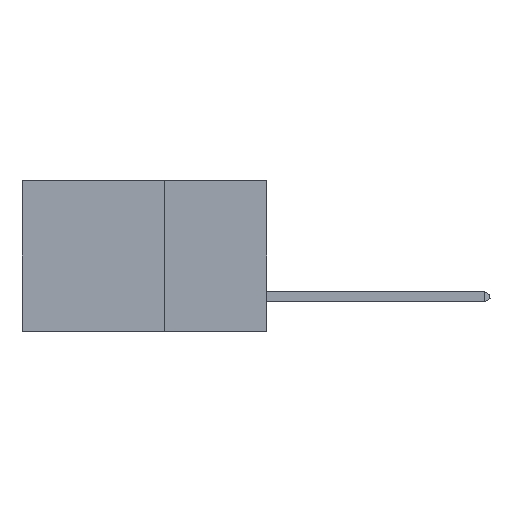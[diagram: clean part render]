
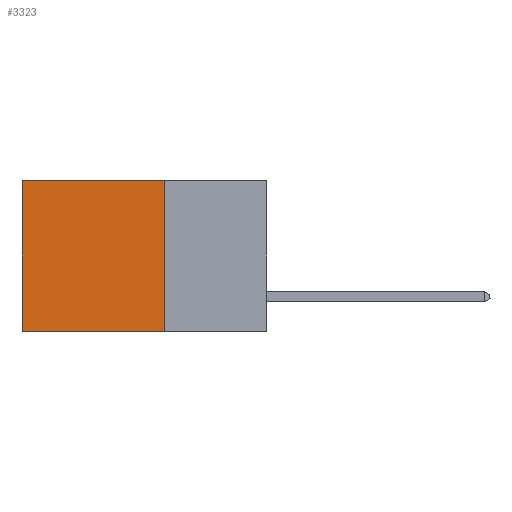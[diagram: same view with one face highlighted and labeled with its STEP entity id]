
A CAD part, left-side view. The second image highlights one B-rep face of the part: STEP entity #3323.
In plain terms, the highlighted planar face has unit normal (-1, 0, 0).
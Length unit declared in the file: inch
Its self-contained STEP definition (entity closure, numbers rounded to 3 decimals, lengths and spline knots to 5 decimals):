
#130 = ORIENTED_EDGE ( 'NONE', *, *, #22767, .F. ) ;
#2065 = CARTESIAN_POINT ( 'NONE',  ( 0.2875, 0.25, 0. ) ) ;
#2497 = DIRECTION ( 'NONE',  ( 0., 1., 0. ) ) ;
#3039 = VERTEX_POINT ( 'NONE', #33966 ) ;
#3323 = ADVANCED_FACE ( 'NONE', ( #24807 ), #29328, .F. ) ;
#4617 = LINE ( 'NONE', #5900, #30110 ) ;
#5057 = ORIENTED_EDGE ( 'NONE', *, *, #29074, .F. ) ;
#5900 = CARTESIAN_POINT ( 'NONE',  ( 0.2875, 0.25, 0. ) ) ;
#6223 = VERTEX_POINT ( 'NONE', #16613 ) ;
#7094 = CARTESIAN_POINT ( 'NONE',  ( 0.2875, 0.25, 0. ) ) ;
#10173 = CARTESIAN_POINT ( 'NONE',  ( 0.2875, 0.6, 0. ) ) ;
#11551 = AXIS2_PLACEMENT_3D ( 'NONE', #29698, #20907, #32664 ) ;
#12199 = LINE ( 'NONE', #32930, #18725 ) ;
#16613 = CARTESIAN_POINT ( 'NONE',  ( 0.2875, 0.6, -0.37 ) ) ;
#18725 = VECTOR ( 'NONE', #32424, 39.37008 ) ;
#19114 = DIRECTION ( 'NONE',  ( 0., 0., -1. ) ) ;
#20099 = LINE ( 'NONE', #2065, #28431 ) ;
#20907 = DIRECTION ( 'NONE',  ( 1., 0., 0. ) ) ;
#22478 = CARTESIAN_POINT ( 'NONE',  ( 0.2875, 0.6, 0. ) ) ;
#22767 = EDGE_CURVE ( 'NONE', #35530, #3039, #20099, .T. ) ;
#24807 = FACE_OUTER_BOUND ( 'NONE', #32636, .T. ) ;
#24837 = VECTOR ( 'NONE', #19114, 39.37008 ) ;
#25756 = LINE ( 'NONE', #10173, #24837 ) ;
#28431 = VECTOR ( 'NONE', #37460, 39.37008 ) ;
#29074 = EDGE_CURVE ( 'NONE', #3039, #6223, #12199, .T. ) ;
#29328 = PLANE ( 'NONE',  #11551 ) ;
#29698 = CARTESIAN_POINT ( 'NONE',  ( 0.2875, 0.25, 0. ) ) ;
#30110 = VECTOR ( 'NONE', #2497, 39.37008 ) ;
#30377 = EDGE_CURVE ( 'NONE', #35530, #37483, #4617, .T. ) ;
#32370 = EDGE_CURVE ( 'NONE', #37483, #6223, #25756, .T. ) ;
#32424 = DIRECTION ( 'NONE',  ( 0., 1., 0. ) ) ;
#32636 = EDGE_LOOP ( 'NONE', ( #33134, #5057, #130, #35337 ) ) ;
#32664 = DIRECTION ( 'NONE',  ( 0., 0., -1. ) ) ;
#32930 = CARTESIAN_POINT ( 'NONE',  ( 0.2875, 0.25, -0.37 ) ) ;
#33134 = ORIENTED_EDGE ( 'NONE', *, *, #32370, .T. ) ;
#33966 = CARTESIAN_POINT ( 'NONE',  ( 0.2875, 0.25, -0.37 ) ) ;
#35337 = ORIENTED_EDGE ( 'NONE', *, *, #30377, .T. ) ;
#35530 = VERTEX_POINT ( 'NONE', #7094 ) ;
#37460 = DIRECTION ( 'NONE',  ( 0., 0., -1. ) ) ;
#37483 = VERTEX_POINT ( 'NONE', #22478 ) ;
